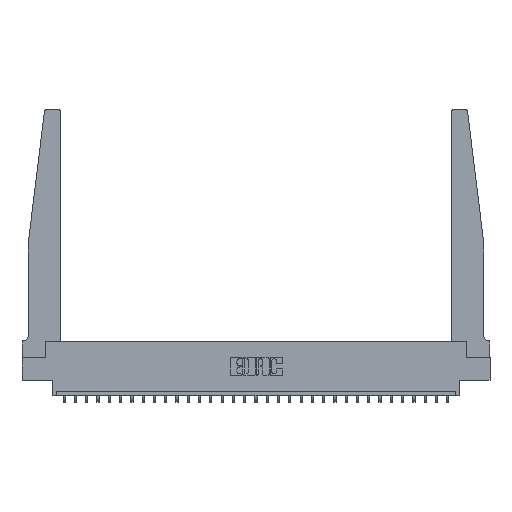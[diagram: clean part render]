
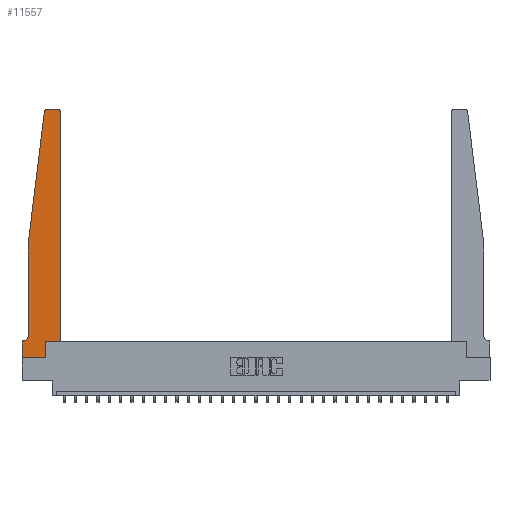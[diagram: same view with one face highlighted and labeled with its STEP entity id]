
A CAD part, top view. The second image highlights one B-rep face of the part: STEP entity #11557.
In plain terms, the highlighted planar face has unit normal (0, 0, 1).
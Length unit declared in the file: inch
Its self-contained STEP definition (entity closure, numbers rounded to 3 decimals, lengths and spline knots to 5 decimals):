
#40 = CARTESIAN_POINT ( 'NONE',  ( 0., 0., 0.37 ) ) ;
#122 = LINE ( 'NONE', #40, #5851 ) ;
#361 = DIRECTION ( 'NONE',  ( 0., 0., -1. ) ) ;
#1489 = CARTESIAN_POINT ( 'NONE',  ( 0.27653, 2.72, 0.37 ) ) ;
#1849 = EDGE_CURVE ( 'NONE', #4201, #8978, #20292, .T. ) ;
#2153 = EDGE_CURVE ( 'NONE', #8978, #16507, #18647, .T. ) ;
#3096 = FACE_OUTER_BOUND ( 'NONE', #13438, .T. ) ;
#3647 = DIRECTION ( 'NONE',  ( 1., 0., 0. ) ) ;
#3667 = EDGE_CURVE ( 'NONE', #24516, #18748, #122, .T. ) ;
#3821 = CARTESIAN_POINT ( 'NONE',  ( 0.2605, 0., 0.37 ) ) ;
#3929 = CARTESIAN_POINT ( 'NONE',  ( 0.065, 0.2375, 0.37 ) ) ;
#4201 = VERTEX_POINT ( 'NONE', #17164 ) ;
#4488 = CIRCLE ( 'NONE', #16086, 0.03 ) ;
#4525 = DIRECTION ( 'NONE',  ( 0., 0., 1. ) ) ;
#4550 = CARTESIAN_POINT ( 'NONE',  ( 0.425, 0.18, 0.37 ) ) ;
#5844 = ORIENTED_EDGE ( 'NONE', *, *, #9035, .T. ) ;
#5851 = VECTOR ( 'NONE', #12913, 39.37008 ) ;
#6569 = VECTOR ( 'NONE', #12815, 39.37008 ) ;
#6706 = CIRCLE ( 'NONE', #18453, 0.05 ) ;
#6907 = ORIENTED_EDGE ( 'NONE', *, *, #14240, .T. ) ;
#7227 = ORIENTED_EDGE ( 'NONE', *, *, #17803, .T. ) ;
#7401 = ORIENTED_EDGE ( 'NONE', *, *, #11081, .T. ) ;
#7981 = PLANE ( 'NONE',  #22643 ) ;
#8077 = CARTESIAN_POINT ( 'NONE',  ( 0., 0.1875, 0.37 ) ) ;
#8719 = CIRCLE ( 'NONE', #25018, 0.03 ) ;
#8905 = VECTOR ( 'NONE', #14252, 39.37008 ) ;
#8978 = VERTEX_POINT ( 'NONE', #18174 ) ;
#9035 = EDGE_CURVE ( 'NONE', #11996, #16254, #14977, .T. ) ;
#9337 = CARTESIAN_POINT ( 'NONE',  ( 0.27653, 2.75, 0.37 ) ) ;
#9865 = CARTESIAN_POINT ( 'NONE',  ( 0.425, 0.18, 0.37 ) ) ;
#10042 = VECTOR ( 'NONE', #17452, 39.37008 ) ;
#10233 = DIRECTION ( 'NONE',  ( 1., 0., 0. ) ) ;
#10607 = CARTESIAN_POINT ( 'NONE',  ( 0.065, 1.25, 0.37 ) ) ;
#10862 = VERTEX_POINT ( 'NONE', #18994 ) ;
#11081 = EDGE_CURVE ( 'NONE', #10862, #20081, #4488, .T. ) ;
#11148 = VERTEX_POINT ( 'NONE', #21732 ) ;
#11557 = ADVANCED_FACE ( 'NONE', ( #3096 ), #7981, .T. ) ;
#11996 = VERTEX_POINT ( 'NONE', #12073 ) ;
#12020 = DIRECTION ( 'NONE',  ( 1., 0., 0. ) ) ;
#12073 = CARTESIAN_POINT ( 'NONE',  ( 0.2605, 0.18, 0.37 ) ) ;
#12718 = CARTESIAN_POINT ( 'NONE',  ( 0.395, 2.75, 0.37 ) ) ;
#12755 = DIRECTION ( 'NONE',  ( 0., -1., 0. ) ) ;
#12815 = DIRECTION ( 'NONE',  ( -1., 0., 0. ) ) ;
#12913 = DIRECTION ( 'NONE',  ( 1., 0., 0. ) ) ;
#12995 = VECTOR ( 'NONE', #12755, 39.37008 ) ;
#13228 = CARTESIAN_POINT ( 'NONE',  ( 0.015, 0.2375, 0.37 ) ) ;
#13342 = DIRECTION ( 'NONE',  ( 0., 1., 0. ) ) ;
#13438 = EDGE_LOOP ( 'NONE', ( #19338, #14789, #20175, #18025, #6907, #25785, #22090, #21023, #7227, #5844, #14529, #7401 ) ) ;
#13659 = VECTOR ( 'NONE', #21380, 39.37008 ) ;
#13846 = CARTESIAN_POINT ( 'NONE',  ( 0.065, 1.25, 0.37 ) ) ;
#14240 = EDGE_CURVE ( 'NONE', #16507, #17486, #6706, .T. ) ;
#14252 = DIRECTION ( 'NONE',  ( -1., 0., 0. ) ) ;
#14325 = LINE ( 'NONE', #25563, #13659 ) ;
#14529 = ORIENTED_EDGE ( 'NONE', *, *, #20240, .T. ) ;
#14575 = EDGE_CURVE ( 'NONE', #24433, #4201, #8719, .T. ) ;
#14789 = ORIENTED_EDGE ( 'NONE', *, *, #14575, .T. ) ;
#14945 = CARTESIAN_POINT ( 'NONE',  ( 0.065, 0.1875, 0.37 ) ) ;
#14977 = LINE ( 'NONE', #9865, #26247 ) ;
#15237 = VECTOR ( 'NONE', #13342, 39.37008 ) ;
#15323 = VECTOR ( 'NONE', #20161, 39.37008 ) ;
#15355 = DIRECTION ( 'NONE',  ( -1., 0., 0. ) ) ;
#15683 = LINE ( 'NONE', #4550, #10042 ) ;
#15906 = CARTESIAN_POINT ( 'NONE',  ( 0.425, 0.18, 0.37 ) ) ;
#16086 = AXIS2_PLACEMENT_3D ( 'NONE', #17334, #4525, #19453 ) ;
#16254 = VERTEX_POINT ( 'NONE', #15906 ) ;
#16481 = DIRECTION ( 'NONE',  ( 0., 0., 1. ) ) ;
#16507 = VERTEX_POINT ( 'NONE', #3929 ) ;
#17164 = CARTESIAN_POINT ( 'NONE',  ( 0.24675, 2.72367, 0.37 ) ) ;
#17334 = CARTESIAN_POINT ( 'NONE',  ( 0.395, 2.72, 0.37 ) ) ;
#17452 = DIRECTION ( 'NONE',  ( 0., 1., 0. ) ) ;
#17486 = VERTEX_POINT ( 'NONE', #18768 ) ;
#17803 = EDGE_CURVE ( 'NONE', #18748, #11996, #20882, .T. ) ;
#17940 = LINE ( 'NONE', #14945, #6569 ) ;
#18025 = ORIENTED_EDGE ( 'NONE', *, *, #2153, .T. ) ;
#18174 = CARTESIAN_POINT ( 'NONE',  ( 0.065, 1.25, 0.37 ) ) ;
#18453 = AXIS2_PLACEMENT_3D ( 'NONE', #13228, #361, #15355 ) ;
#18647 = LINE ( 'NONE', #10607, #12995 ) ;
#18748 = VERTEX_POINT ( 'NONE', #3821 ) ;
#18768 = CARTESIAN_POINT ( 'NONE',  ( 0.015, 0.1875, 0.37 ) ) ;
#18994 = CARTESIAN_POINT ( 'NONE',  ( 0.425, 2.72, 0.37 ) ) ;
#19338 = ORIENTED_EDGE ( 'NONE', *, *, #27162, .T. ) ;
#19453 = DIRECTION ( 'NONE',  ( 1., 0., 0. ) ) ;
#20081 = VERTEX_POINT ( 'NONE', #12718 ) ;
#20161 = DIRECTION ( 'NONE',  ( -0.122, -0.992, 0. ) ) ;
#20175 = ORIENTED_EDGE ( 'NONE', *, *, #1849, .T. ) ;
#20194 = CARTESIAN_POINT ( 'NONE',  ( 0., 0., 0.37 ) ) ;
#20240 = EDGE_CURVE ( 'NONE', #16254, #10862, #15683, .T. ) ;
#20292 = LINE ( 'NONE', #13846, #15323 ) ;
#20784 = EDGE_CURVE ( 'NONE', #11148, #24516, #14325, .T. ) ;
#20882 = LINE ( 'NONE', #21761, #15237 ) ;
#21023 = ORIENTED_EDGE ( 'NONE', *, *, #3667, .T. ) ;
#21380 = DIRECTION ( 'NONE',  ( 0., -1., 0. ) ) ;
#21732 = CARTESIAN_POINT ( 'NONE',  ( 0., 0.1875, 0.37 ) ) ;
#21761 = CARTESIAN_POINT ( 'NONE',  ( 0.2605, 0.18, 0.37 ) ) ;
#22090 = ORIENTED_EDGE ( 'NONE', *, *, #20784, .T. ) ;
#22643 = AXIS2_PLACEMENT_3D ( 'NONE', #8077, #22938, #10233 ) ;
#22938 = DIRECTION ( 'NONE',  ( 0., 0., 1. ) ) ;
#24433 = VERTEX_POINT ( 'NONE', #9337 ) ;
#24516 = VERTEX_POINT ( 'NONE', #20194 ) ;
#24821 = CARTESIAN_POINT ( 'NONE',  ( 0.25, 2.75, 0.37 ) ) ;
#25018 = AXIS2_PLACEMENT_3D ( 'NONE', #1489, #16481, #3647 ) ;
#25563 = CARTESIAN_POINT ( 'NONE',  ( 0., 0., 0.37 ) ) ;
#25785 = ORIENTED_EDGE ( 'NONE', *, *, #26749, .T. ) ;
#26247 = VECTOR ( 'NONE', #12020, 39.37008 ) ;
#26507 = LINE ( 'NONE', #24821, #8905 ) ;
#26749 = EDGE_CURVE ( 'NONE', #17486, #11148, #17940, .T. ) ;
#27162 = EDGE_CURVE ( 'NONE', #20081, #24433, #26507, .T. ) ;
